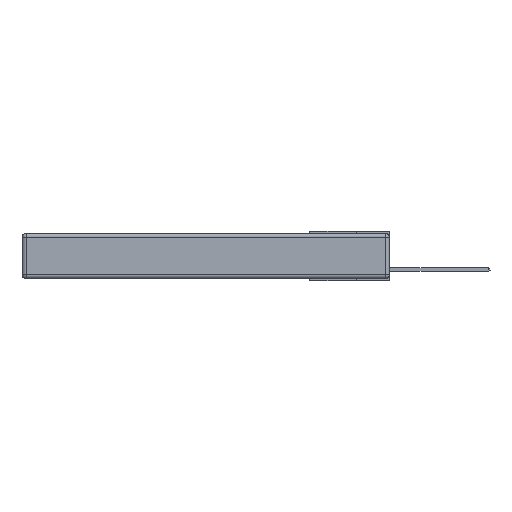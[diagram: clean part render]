
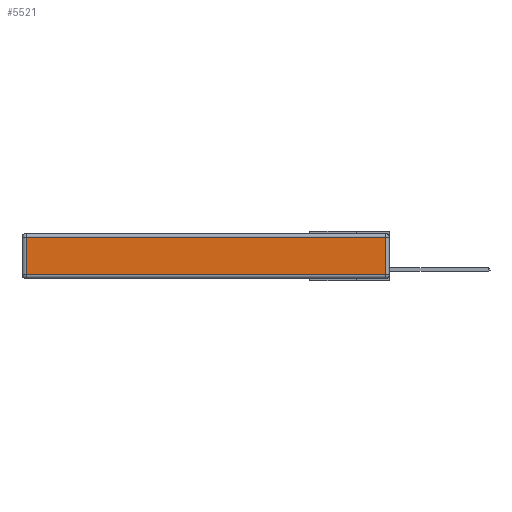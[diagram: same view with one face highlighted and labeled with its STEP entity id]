
A CAD part, left-side view. The second image highlights one B-rep face of the part: STEP entity #5521.
In plain terms, the highlighted planar face has unit normal (-1, 0, 0).
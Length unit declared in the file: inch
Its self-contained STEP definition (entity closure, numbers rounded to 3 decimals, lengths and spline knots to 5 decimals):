
#850 = EDGE_CURVE ( 'NONE', #21576, #24429, #24794, .T. ) ;
#879 = ORIENTED_EDGE ( 'NONE', *, *, #5951, .T. ) ;
#1654 = FACE_OUTER_BOUND ( 'NONE', #9887, .T. ) ;
#1982 = VECTOR ( 'NONE', #11664, 39.37008 ) ;
#2105 = DIRECTION ( 'NONE',  ( 0., 0., 1. ) ) ;
#2382 = VERTEX_POINT ( 'NONE', #8017 ) ;
#3613 = VECTOR ( 'NONE', #22778, 39.37008 ) ;
#4487 = ORIENTED_EDGE ( 'NONE', *, *, #4526, .T. ) ;
#4526 = EDGE_CURVE ( 'NONE', #24429, #18397, #6773, .T. ) ;
#4550 = CARTESIAN_POINT ( 'NONE',  ( 0., 2.72, -0.03 ) ) ;
#5521 = ADVANCED_FACE ( 'NONE', ( #1654 ), #7806, .T. ) ;
#5694 = AXIS2_PLACEMENT_3D ( 'NONE', #11881, #17718, #15902 ) ;
#5951 = EDGE_CURVE ( 'NONE', #2382, #21576, #19924, .T. ) ;
#6773 = LINE ( 'NONE', #25294, #3613 ) ;
#7806 = PLANE ( 'NONE',  #5694 ) ;
#7939 = CARTESIAN_POINT ( 'NONE',  ( 0., 0.03, -0.313 ) ) ;
#7985 = LINE ( 'NONE', #15694, #1982 ) ;
#8017 = CARTESIAN_POINT ( 'NONE',  ( 0., 2.72, -0.313 ) ) ;
#9212 = CARTESIAN_POINT ( 'NONE',  ( 0., 0., -0.313 ) ) ;
#9887 = EDGE_LOOP ( 'NONE', ( #879, #11591, #4487, #26018 ) ) ;
#11591 = ORIENTED_EDGE ( 'NONE', *, *, #850, .T. ) ;
#11664 = DIRECTION ( 'NONE',  ( 0., 0., -1. ) ) ;
#11881 = CARTESIAN_POINT ( 'NONE',  ( 0., 0., -0.343 ) ) ;
#14156 = CARTESIAN_POINT ( 'NONE',  ( 0., 0.03, -0.03 ) ) ;
#15694 = CARTESIAN_POINT ( 'NONE',  ( 0., 2.72, -0.343 ) ) ;
#15902 = DIRECTION ( 'NONE',  ( 0., 0., 1. ) ) ;
#17325 = DIRECTION ( 'NONE',  ( 0., -1., 0. ) ) ;
#17718 = DIRECTION ( 'NONE',  ( -1., 0., 0. ) ) ;
#18397 = VERTEX_POINT ( 'NONE', #4550 ) ;
#18834 = VECTOR ( 'NONE', #2105, 39.37008 ) ;
#19924 = LINE ( 'NONE', #9212, #20881 ) ;
#20337 = CARTESIAN_POINT ( 'NONE',  ( 0., 0.03, -0.343 ) ) ;
#20881 = VECTOR ( 'NONE', #17325, 39.37008 ) ;
#21576 = VERTEX_POINT ( 'NONE', #7939 ) ;
#22778 = DIRECTION ( 'NONE',  ( 0., 1., 0. ) ) ;
#24429 = VERTEX_POINT ( 'NONE', #14156 ) ;
#24794 = LINE ( 'NONE', #20337, #18834 ) ;
#25294 = CARTESIAN_POINT ( 'NONE',  ( 0., 2.75, -0.03 ) ) ;
#25373 = EDGE_CURVE ( 'NONE', #18397, #2382, #7985, .T. ) ;
#26018 = ORIENTED_EDGE ( 'NONE', *, *, #25373, .T. ) ;
